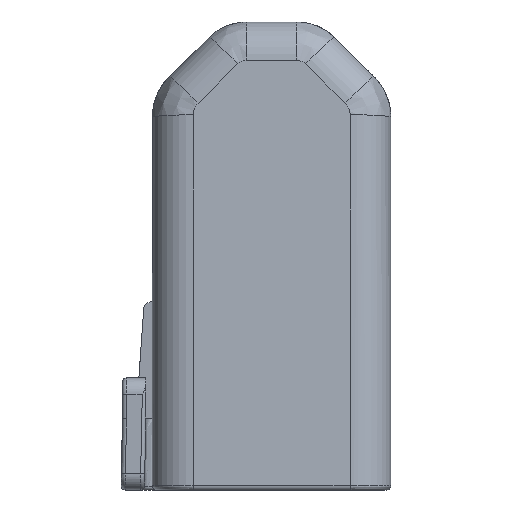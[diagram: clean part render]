
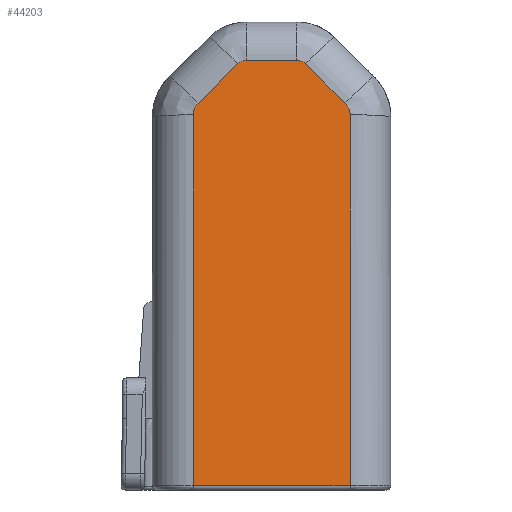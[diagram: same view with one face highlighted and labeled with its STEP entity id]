
A CAD part, front view. The second image highlights one B-rep face of the part: STEP entity #44203.
In plain terms, the highlighted planar face has unit normal (0, -0.998, 0.062).
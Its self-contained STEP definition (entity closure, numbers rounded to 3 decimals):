
#2800=ELLIPSE('',#45766,2.004,2.);
#2801=ELLIPSE('',#45770,1.503,1.5);
#2802=ELLIPSE('',#45774,1.503,1.5);
#2803=ELLIPSE('',#45778,2.004,2.);
#7738=FACE_OUTER_BOUND('',#10352,.T.);
#10352=EDGE_LOOP('',(#40686,#40687,#40688,#40689,#40690,#40691,#40692,#40693,
#40694,#40695));
#13483=LINE('',#87951,#16657);
#13537=LINE('',#88581,#16711);
#13538=LINE('',#88613,#16712);
#13539=LINE('',#88644,#16713);
#13540=LINE('',#88675,#16714);
#13541=LINE('',#88704,#16715);
#16657=VECTOR('',#51623,10.);
#16711=VECTOR('',#51913,10.);
#16712=VECTOR('',#51924,10.);
#16713=VECTOR('',#51933,10.);
#16714=VECTOR('',#51942,10.);
#16715=VECTOR('',#51949,10.);
#21035=VERTEX_POINT('',#87943);
#21037=VERTEX_POINT('',#87949);
#21101=VERTEX_POINT('',#88580);
#21102=VERTEX_POINT('',#88607);
#21103=VERTEX_POINT('',#88611);
#21104=VERTEX_POINT('',#88638);
#21105=VERTEX_POINT('',#88642);
#21106=VERTEX_POINT('',#88669);
#21107=VERTEX_POINT('',#88673);
#21108=VERTEX_POINT('',#88700);
#27537=EDGE_CURVE('',#21037,#21035,#13483,.T.);
#27670=EDGE_CURVE('',#21035,#21101,#13537,.T.);
#27673=EDGE_CURVE('',#21101,#21102,#2800,.T.);
#27675=EDGE_CURVE('',#21102,#21103,#13538,.T.);
#27677=EDGE_CURVE('',#21103,#21104,#2801,.T.);
#27679=EDGE_CURVE('',#21104,#21105,#13539,.T.);
#27681=EDGE_CURVE('',#21105,#21106,#2802,.T.);
#27683=EDGE_CURVE('',#21106,#21107,#13540,.T.);
#27685=EDGE_CURVE('',#21107,#21108,#2803,.T.);
#27686=EDGE_CURVE('',#21108,#21037,#13541,.T.);
#40686=ORIENTED_EDGE('',*,*,#27537,.F.);
#40687=ORIENTED_EDGE('',*,*,#27686,.F.);
#40688=ORIENTED_EDGE('',*,*,#27685,.F.);
#40689=ORIENTED_EDGE('',*,*,#27683,.F.);
#40690=ORIENTED_EDGE('',*,*,#27681,.F.);
#40691=ORIENTED_EDGE('',*,*,#27679,.F.);
#40692=ORIENTED_EDGE('',*,*,#27677,.F.);
#40693=ORIENTED_EDGE('',*,*,#27675,.F.);
#40694=ORIENTED_EDGE('',*,*,#27673,.F.);
#40695=ORIENTED_EDGE('',*,*,#27670,.F.);
#41806=PLANE('',#45780);
#44203=ADVANCED_FACE('',(#7738),#41806,.F.);
#45766=AXIS2_PLACEMENT_3D('',#88609,#51918,#51919);
#45770=AXIS2_PLACEMENT_3D('',#88640,#51927,#51928);
#45774=AXIS2_PLACEMENT_3D('',#88671,#51936,#51937);
#45778=AXIS2_PLACEMENT_3D('',#88702,#51945,#51946);
#45780=AXIS2_PLACEMENT_3D('',#88705,#51950,#51951);
#51623=DIRECTION('',(-1.,0.,0.));
#51913=DIRECTION('',(0.,0.062,0.998));
#51918=DIRECTION('center_axis',(0.,0.998,-0.062));
#51919=DIRECTION('ref_axis',(0.,0.062,0.998));
#51924=DIRECTION('',(0.711,0.044,0.701));
#51927=DIRECTION('center_axis',(0.,0.998,-0.062));
#51928=DIRECTION('ref_axis',(0.,0.062,0.998));
#51933=DIRECTION('',(1.,0.,0.));
#51936=DIRECTION('center_axis',(0.,0.998,-0.062));
#51937=DIRECTION('ref_axis',(0.,0.062,0.998));
#51942=DIRECTION('',(0.71,-0.044,-0.703));
#51945=DIRECTION('center_axis',(0.,0.998,-0.062));
#51946=DIRECTION('ref_axis',(0.,0.062,0.998));
#51949=DIRECTION('',(0.,-0.062,-0.998));
#51950=DIRECTION('center_axis',(0.,0.998,-0.062));
#51951=DIRECTION('ref_axis',(0.,0.062,0.998));
#87943=CARTESIAN_POINT('',(-113.44,-42.233,-15.728));
#87949=CARTESIAN_POINT('',(-94.223,-42.233,-15.728));
#87951=CARTESIAN_POINT('',(-111.72,-42.233,-15.728));
#88580=CARTESIAN_POINT('',(-113.44,-39.408,29.683));
#88581=CARTESIAN_POINT('',(-113.44,-41.432,-2.846));
#88607=CARTESIAN_POINT('',(-112.844,-39.32,31.107));
#88609=CARTESIAN_POINT('Origin',(-111.44,-39.408,29.683));
#88611=CARTESIAN_POINT('',(-107.954,-39.02,35.929));
#88613=CARTESIAN_POINT('',(-126.468,-40.155,17.673));
#88638=CARTESIAN_POINT('',(-106.9,-38.993,36.361));
#88640=CARTESIAN_POINT('Origin',(-106.9,-39.086,34.861));
#88642=CARTESIAN_POINT('',(-100.738,-38.993,36.361));
#88644=CARTESIAN_POINT('',(-112.67,-38.993,36.361));
#88669=CARTESIAN_POINT('',(-99.683,-39.02,35.927));
#88671=CARTESIAN_POINT('Origin',(-100.738,-39.086,34.861));
#88673=CARTESIAN_POINT('',(-94.817,-39.319,31.111));
#88675=CARTESIAN_POINT('',(-90.992,-39.555,27.327));
#88700=CARTESIAN_POINT('',(-94.223,-39.408,29.69));
#88702=CARTESIAN_POINT('Origin',(-96.223,-39.408,29.69));
#88704=CARTESIAN_POINT('',(-94.223,-37.331,63.082));
#88705=CARTESIAN_POINT('Origin',(-118.44,-42.266,-16.259));
